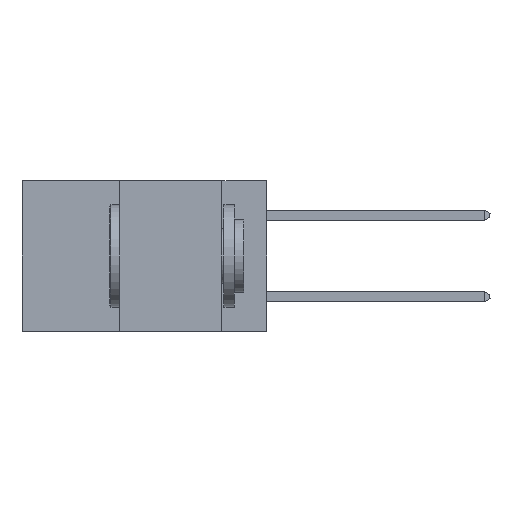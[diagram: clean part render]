
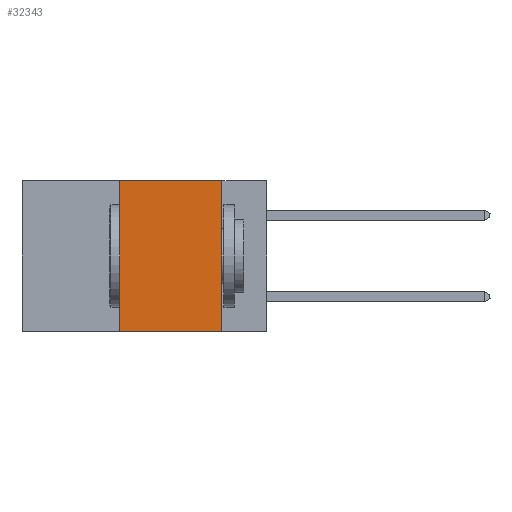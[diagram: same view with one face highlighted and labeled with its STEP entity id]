
A CAD part, left-side view. The second image highlights one B-rep face of the part: STEP entity #32343.
In plain terms, the highlighted planar face has unit normal (-1, 0, 0).
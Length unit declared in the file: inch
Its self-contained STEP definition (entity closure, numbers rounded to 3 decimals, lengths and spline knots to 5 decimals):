
#474 = ORIENTED_EDGE ( 'NONE', *, *, #3246, .F. ) ;
#644 = VERTEX_POINT ( 'NONE', #7569 ) ;
#1005 = LINE ( 'NONE', #8177, #36238 ) ;
#1350 = CARTESIAN_POINT ( 'NONE',  ( 0., 0.36, 0. ) ) ;
#3198 = PLANE ( 'NONE',  #18998 ) ;
#3238 = CARTESIAN_POINT ( 'NONE',  ( 0., 0.36, -0.37 ) ) ;
#3246 = EDGE_CURVE ( 'NONE', #20611, #33043, #29689, .T. ) ;
#3638 = VECTOR ( 'NONE', #20103, 39.37008 ) ;
#5693 = VECTOR ( 'NONE', #17249, 39.37008 ) ;
#7569 = CARTESIAN_POINT ( 'NONE',  ( 0., 0.11, 0. ) ) ;
#8055 = ORIENTED_EDGE ( 'NONE', *, *, #18136, .T. ) ;
#8177 = CARTESIAN_POINT ( 'NONE',  ( 0., 0.6, 0. ) ) ;
#9630 = DIRECTION ( 'NONE',  ( 1., 0., 0. ) ) ;
#13051 = DIRECTION ( 'NONE',  ( 0., 0., -1. ) ) ;
#17249 = DIRECTION ( 'NONE',  ( 0., -1., 0. ) ) ;
#18136 = EDGE_CURVE ( 'NONE', #20611, #40814, #24925, .T. ) ;
#18998 = AXIS2_PLACEMENT_3D ( 'NONE', #37232, #9630, #13051 ) ;
#20103 = DIRECTION ( 'NONE',  ( 0., 0., -1. ) ) ;
#20180 = EDGE_CURVE ( 'NONE', #33043, #644, #1005, .T. ) ;
#20497 = EDGE_CURVE ( 'NONE', #644, #40814, #27638, .T. ) ;
#20611 = VERTEX_POINT ( 'NONE', #3238 ) ;
#20639 = VECTOR ( 'NONE', #32040, 39.37008 ) ;
#21587 = ORIENTED_EDGE ( 'NONE', *, *, #20180, .F. ) ;
#24925 = LINE ( 'NONE', #37681, #5693 ) ;
#25477 = DIRECTION ( 'NONE',  ( 0., -1., 0. ) ) ;
#27638 = LINE ( 'NONE', #40453, #3638 ) ;
#29565 = EDGE_LOOP ( 'NONE', ( #32905, #21587, #474, #8055 ) ) ;
#29689 = LINE ( 'NONE', #1350, #20639 ) ;
#32040 = DIRECTION ( 'NONE',  ( 0., 0., 1. ) ) ;
#32343 = ADVANCED_FACE ( 'NONE', ( #34790 ), #3198, .F. ) ;
#32905 = ORIENTED_EDGE ( 'NONE', *, *, #20497, .F. ) ;
#33043 = VERTEX_POINT ( 'NONE', #34169 ) ;
#34169 = CARTESIAN_POINT ( 'NONE',  ( 0., 0.36, 0. ) ) ;
#34790 = FACE_OUTER_BOUND ( 'NONE', #29565, .T. ) ;
#36238 = VECTOR ( 'NONE', #25477, 39.37008 ) ;
#37232 = CARTESIAN_POINT ( 'NONE',  ( 0., 0.6, 0. ) ) ;
#37681 = CARTESIAN_POINT ( 'NONE',  ( 0., 0.6, -0.37 ) ) ;
#40453 = CARTESIAN_POINT ( 'NONE',  ( 0., 0.11, 0. ) ) ;
#40814 = VERTEX_POINT ( 'NONE', #42150 ) ;
#42150 = CARTESIAN_POINT ( 'NONE',  ( 0., 0.11, -0.37 ) ) ;
